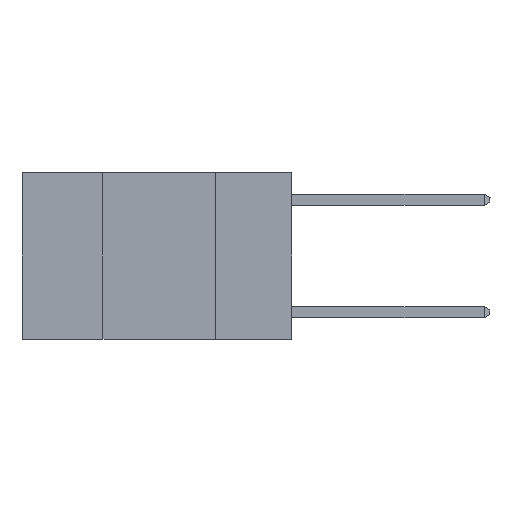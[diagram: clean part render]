
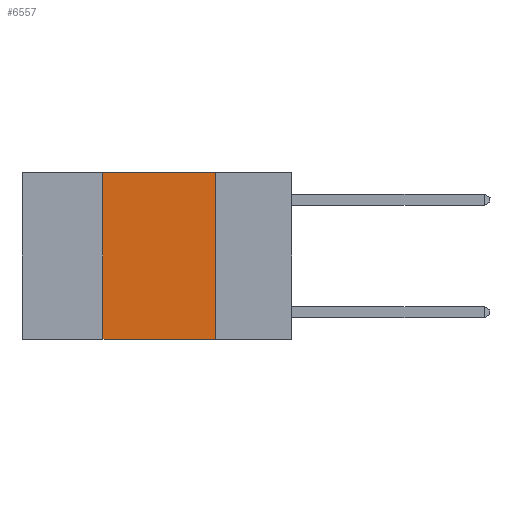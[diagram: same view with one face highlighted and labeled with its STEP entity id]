
A CAD part, left-side view. The second image highlights one B-rep face of the part: STEP entity #6557.
In plain terms, the highlighted planar face has unit normal (-1, 0, 0).
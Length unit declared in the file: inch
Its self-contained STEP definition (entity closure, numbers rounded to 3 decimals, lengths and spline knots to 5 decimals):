
#86 = ORIENTED_EDGE ( 'NONE', *, *, #4929, .F. ) ;
#541 = CARTESIAN_POINT ( 'NONE',  ( 0., 0.17, 0. ) ) ;
#671 = EDGE_LOOP ( 'NONE', ( #9307, #7170, #86, #6834 ) ) ;
#734 = LINE ( 'NONE', #541, #7352 ) ;
#1209 = VECTOR ( 'NONE', #10345, 39.37008 ) ;
#1252 = CARTESIAN_POINT ( 'NONE',  ( 0., 0.6, 0. ) ) ;
#2092 = EDGE_CURVE ( 'NONE', #4776, #3657, #10243, .T. ) ;
#2194 = CARTESIAN_POINT ( 'NONE',  ( 0., 0.6, 0. ) ) ;
#2606 = EDGE_CURVE ( 'NONE', #3657, #3637, #734, .T. ) ;
#2907 = AXIS2_PLACEMENT_3D ( 'NONE', #2194, #3828, #3670 ) ;
#3258 = CARTESIAN_POINT ( 'NONE',  ( 0., 0.17, -0.37 ) ) ;
#3308 = CARTESIAN_POINT ( 'NONE',  ( 0., 0.17, 0. ) ) ;
#3637 = VERTEX_POINT ( 'NONE', #3258 ) ;
#3657 = VERTEX_POINT ( 'NONE', #3308 ) ;
#3670 = DIRECTION ( 'NONE',  ( 0., 0., -1. ) ) ;
#3828 = DIRECTION ( 'NONE',  ( 1., 0., 0. ) ) ;
#3866 = EDGE_CURVE ( 'NONE', #9167, #3637, #6865, .T. ) ;
#4041 = DIRECTION ( 'NONE',  ( 0., 0., 1. ) ) ;
#4776 = VERTEX_POINT ( 'NONE', #8740 ) ;
#4929 = EDGE_CURVE ( 'NONE', #9167, #4776, #6572, .T. ) ;
#5664 = VECTOR ( 'NONE', #4041, 39.37008 ) ;
#6409 = DIRECTION ( 'NONE',  ( 0., 0., -1. ) ) ;
#6557 = ADVANCED_FACE ( 'NONE', ( #9485 ), #7870, .F. ) ;
#6572 = LINE ( 'NONE', #8085, #5664 ) ;
#6834 = ORIENTED_EDGE ( 'NONE', *, *, #3866, .T. ) ;
#6865 = LINE ( 'NONE', #9681, #8322 ) ;
#7014 = CARTESIAN_POINT ( 'NONE',  ( 0., 0.42, -0.37 ) ) ;
#7170 = ORIENTED_EDGE ( 'NONE', *, *, #2092, .F. ) ;
#7352 = VECTOR ( 'NONE', #6409, 39.37008 ) ;
#7870 = PLANE ( 'NONE',  #2907 ) ;
#8085 = CARTESIAN_POINT ( 'NONE',  ( 0., 0.42, 0. ) ) ;
#8322 = VECTOR ( 'NONE', #10538, 39.37008 ) ;
#8740 = CARTESIAN_POINT ( 'NONE',  ( 0., 0.42, 0. ) ) ;
#9167 = VERTEX_POINT ( 'NONE', #7014 ) ;
#9307 = ORIENTED_EDGE ( 'NONE', *, *, #2606, .F. ) ;
#9485 = FACE_OUTER_BOUND ( 'NONE', #671, .T. ) ;
#9681 = CARTESIAN_POINT ( 'NONE',  ( 0., 0.6, -0.37 ) ) ;
#10243 = LINE ( 'NONE', #1252, #1209 ) ;
#10345 = DIRECTION ( 'NONE',  ( 0., -1., 0. ) ) ;
#10538 = DIRECTION ( 'NONE',  ( 0., -1., 0. ) ) ;
